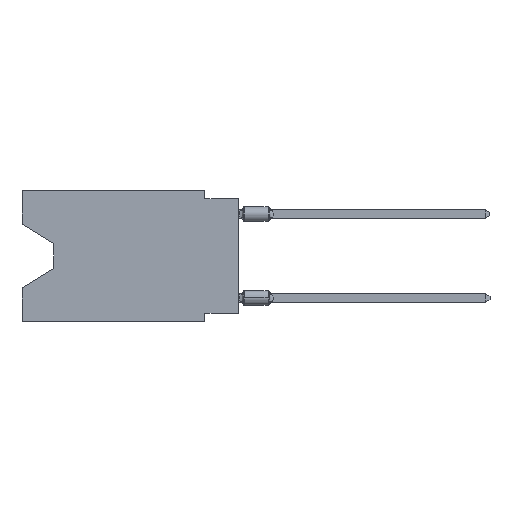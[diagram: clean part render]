
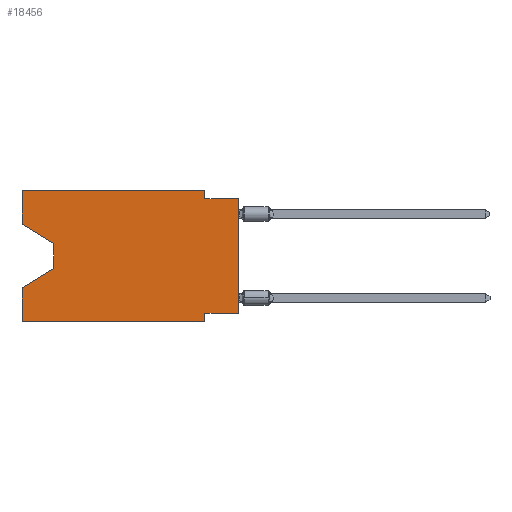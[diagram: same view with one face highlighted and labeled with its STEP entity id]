
A CAD part, left-side view. The second image highlights one B-rep face of the part: STEP entity #18456.
In plain terms, the highlighted planar face has unit normal (-1, 0, 0).
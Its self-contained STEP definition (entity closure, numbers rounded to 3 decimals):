
#99 = CARTESIAN_POINT ( 'NONE',  ( 0., 16.383, -9.906 ) ) ;
#407 = PLANE ( 'NONE',  #11718 ) ;
#1598 = EDGE_CURVE ( 'NONE', #19317, #12227, #22354, .T. ) ;
#2213 = LINE ( 'NONE', #4374, #3385 ) ;
#2420 = DIRECTION ( 'NONE',  ( 0., 0., -1. ) ) ;
#2675 = LINE ( 'NONE', #99, #5718 ) ;
#2809 = CARTESIAN_POINT ( 'NONE',  ( 0., 16.383, 0. ) ) ;
#2906 = CARTESIAN_POINT ( 'NONE',  ( 0., 16.383, -7.36 ) ) ;
#2950 = VECTOR ( 'NONE', #3378, 1000. ) ;
#2986 = DIRECTION ( 'NONE',  ( 0., 0., -1. ) ) ;
#3033 = EDGE_CURVE ( 'NONE', #22632, #22383, #24503, .T. ) ;
#3378 = DIRECTION ( 'NONE',  ( 0., -1., 0. ) ) ;
#3385 = VECTOR ( 'NONE', #6532, 1000. ) ;
#3674 = DIRECTION ( 'NONE',  ( 0., 0., -1. ) ) ;
#4217 = VERTEX_POINT ( 'NONE', #8173 ) ;
#4374 = CARTESIAN_POINT ( 'NONE',  ( 0., 13.97, -5.893 ) ) ;
#4415 = VECTOR ( 'NONE', #21297, 1000. ) ;
#4537 = ORIENTED_EDGE ( 'NONE', *, *, #3033, .F. ) ;
#4596 = EDGE_CURVE ( 'NONE', #4217, #19110, #15008, .T. ) ;
#4749 = EDGE_CURVE ( 'NONE', #9968, #10474, #6848, .T. ) ;
#4830 = EDGE_CURVE ( 'NONE', #15603, #22632, #9705, .T. ) ;
#5004 = CARTESIAN_POINT ( 'NONE',  ( 0., 2.54, -9.906 ) ) ;
#5092 = DIRECTION ( 'NONE',  ( 0., 0., 1. ) ) ;
#5148 = DIRECTION ( 'NONE',  ( 0., 1., 0. ) ) ;
#5272 = ORIENTED_EDGE ( 'NONE', *, *, #19131, .T. ) ;
#5718 = VECTOR ( 'NONE', #19903, 1000. ) ;
#6076 = VERTEX_POINT ( 'NONE', #18582 ) ;
#6381 = DIRECTION ( 'NONE',  ( 0., -0.855, -0.519 ) ) ;
#6532 = DIRECTION ( 'NONE',  ( 0., 0.855, -0.519 ) ) ;
#6848 = LINE ( 'NONE', #15594, #2950 ) ;
#6895 = LINE ( 'NONE', #5004, #21734 ) ;
#7449 = ORIENTED_EDGE ( 'NONE', *, *, #4749, .F. ) ;
#7495 = ORIENTED_EDGE ( 'NONE', *, *, #4830, .F. ) ;
#7695 = VECTOR ( 'NONE', #13327, 1000. ) ;
#7711 = ORIENTED_EDGE ( 'NONE', *, *, #26675, .T. ) ;
#8173 = CARTESIAN_POINT ( 'NONE',  ( 0., 13.97, -4.013 ) ) ;
#8257 = LINE ( 'NONE', #10556, #4415 ) ;
#8688 = LINE ( 'NONE', #15138, #28382 ) ;
#8763 = CARTESIAN_POINT ( 'NONE',  ( 0., 16.383, 0. ) ) ;
#9184 = DIRECTION ( 'NONE',  ( 0., 0., 1. ) ) ;
#9705 = LINE ( 'NONE', #2809, #17624 ) ;
#9968 = VERTEX_POINT ( 'NONE', #17804 ) ;
#10474 = VERTEX_POINT ( 'NONE', #13701 ) ;
#10556 = CARTESIAN_POINT ( 'NONE',  ( 0., 0., 0. ) ) ;
#11718 = AXIS2_PLACEMENT_3D ( 'NONE', #24381, #19655, #2420 ) ;
#12172 = ORIENTED_EDGE ( 'NONE', *, *, #21084, .F. ) ;
#12227 = VERTEX_POINT ( 'NONE', #2906 ) ;
#12914 = ORIENTED_EDGE ( 'NONE', *, *, #23270, .F. ) ;
#13056 = CARTESIAN_POINT ( 'NONE',  ( 0., 2.54, -9.271 ) ) ;
#13327 = DIRECTION ( 'NONE',  ( 0., -1., 0. ) ) ;
#13406 = CARTESIAN_POINT ( 'NONE',  ( 0., 2.54, 0. ) ) ;
#13701 = CARTESIAN_POINT ( 'NONE',  ( 0., 0., -0.635 ) ) ;
#14186 = EDGE_CURVE ( 'NONE', #19110, #12227, #2213, .T. ) ;
#14412 = VERTEX_POINT ( 'NONE', #13056 ) ;
#14561 = EDGE_CURVE ( 'NONE', #14412, #6076, #6895, .T. ) ;
#14574 = VERTEX_POINT ( 'NONE', #15774 ) ;
#15008 = LINE ( 'NONE', #17163, #24507 ) ;
#15138 = CARTESIAN_POINT ( 'NONE',  ( 0., 16.383, -2.546 ) ) ;
#15594 = CARTESIAN_POINT ( 'NONE',  ( 0., 0., -0.635 ) ) ;
#15603 = VERTEX_POINT ( 'NONE', #16113 ) ;
#15645 = ORIENTED_EDGE ( 'NONE', *, *, #1598, .F. ) ;
#15774 = CARTESIAN_POINT ( 'NONE',  ( 0., 0., -9.271 ) ) ;
#16113 = CARTESIAN_POINT ( 'NONE',  ( 0., 16.383, -2.546 ) ) ;
#16583 = CARTESIAN_POINT ( 'NONE',  ( 0., 2.54, 0. ) ) ;
#17163 = CARTESIAN_POINT ( 'NONE',  ( 0., 13.97, -4.013 ) ) ;
#17624 = VECTOR ( 'NONE', #5092, 1000. ) ;
#17804 = CARTESIAN_POINT ( 'NONE',  ( 0., 2.54, -0.635 ) ) ;
#18456 = ADVANCED_FACE ( 'NONE', ( #19929 ), #407, .F. ) ;
#18582 = CARTESIAN_POINT ( 'NONE',  ( 0., 2.54, -9.906 ) ) ;
#19110 = VERTEX_POINT ( 'NONE', #27501 ) ;
#19131 = EDGE_CURVE ( 'NONE', #14574, #10474, #8257, .T. ) ;
#19238 = ORIENTED_EDGE ( 'NONE', *, *, #14561, .F. ) ;
#19317 = VERTEX_POINT ( 'NONE', #25891 ) ;
#19655 = DIRECTION ( 'NONE',  ( 1., 0., 0. ) ) ;
#19903 = DIRECTION ( 'NONE',  ( 0., -1., 0. ) ) ;
#19929 = FACE_OUTER_BOUND ( 'NONE', #21524, .T. ) ;
#20967 = VECTOR ( 'NONE', #9184, 1000. ) ;
#21084 = EDGE_CURVE ( 'NONE', #14574, #14412, #22654, .T. ) ;
#21174 = LINE ( 'NONE', #16583, #23843 ) ;
#21297 = DIRECTION ( 'NONE',  ( 0., 0., 1. ) ) ;
#21323 = DIRECTION ( 'NONE',  ( 0., 0., -1. ) ) ;
#21464 = ORIENTED_EDGE ( 'NONE', *, *, #4596, .T. ) ;
#21524 = EDGE_LOOP ( 'NONE', ( #28235, #21464, #27921, #15645, #7711, #19238, #12172, #5272, #7449, #12914, #4537, #7495 ) ) ;
#21734 = VECTOR ( 'NONE', #2986, 1000. ) ;
#22264 = EDGE_CURVE ( 'NONE', #15603, #4217, #8688, .T. ) ;
#22354 = LINE ( 'NONE', #22504, #20967 ) ;
#22383 = VERTEX_POINT ( 'NONE', #13406 ) ;
#22504 = CARTESIAN_POINT ( 'NONE',  ( 0., 16.383, 0. ) ) ;
#22632 = VERTEX_POINT ( 'NONE', #8763 ) ;
#22654 = LINE ( 'NONE', #24818, #24648 ) ;
#23270 = EDGE_CURVE ( 'NONE', #22383, #9968, #21174, .T. ) ;
#23843 = VECTOR ( 'NONE', #3674, 1000. ) ;
#24381 = CARTESIAN_POINT ( 'NONE',  ( 0., 16.383, 0. ) ) ;
#24503 = LINE ( 'NONE', #26387, #7695 ) ;
#24507 = VECTOR ( 'NONE', #21323, 1000. ) ;
#24648 = VECTOR ( 'NONE', #5148, 1000. ) ;
#24818 = CARTESIAN_POINT ( 'NONE',  ( 0., 0., -9.271 ) ) ;
#25891 = CARTESIAN_POINT ( 'NONE',  ( 0., 16.383, -9.906 ) ) ;
#26387 = CARTESIAN_POINT ( 'NONE',  ( 0., 16.383, 0. ) ) ;
#26675 = EDGE_CURVE ( 'NONE', #19317, #6076, #2675, .T. ) ;
#27501 = CARTESIAN_POINT ( 'NONE',  ( 0., 13.97, -5.893 ) ) ;
#27921 = ORIENTED_EDGE ( 'NONE', *, *, #14186, .T. ) ;
#28235 = ORIENTED_EDGE ( 'NONE', *, *, #22264, .T. ) ;
#28382 = VECTOR ( 'NONE', #6381, 1000. ) ;
